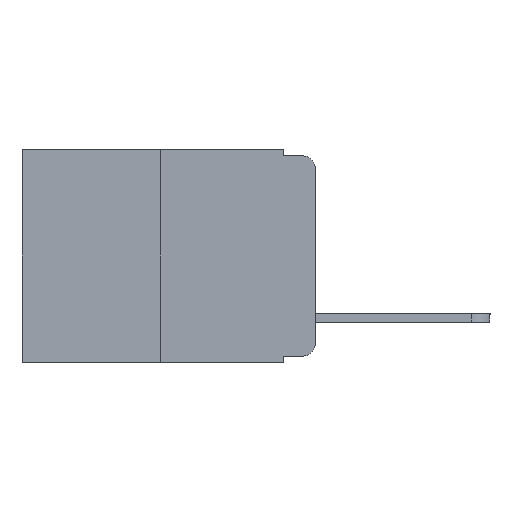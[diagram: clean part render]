
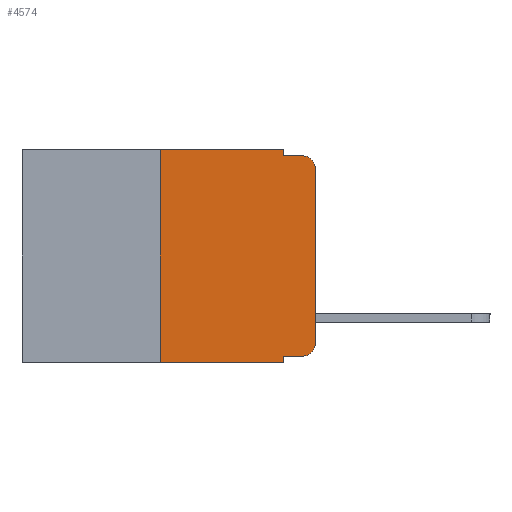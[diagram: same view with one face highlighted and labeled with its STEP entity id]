
A CAD part, left-side view. The second image highlights one B-rep face of the part: STEP entity #4574.
In plain terms, the highlighted planar face has unit normal (-1, 0, 0).
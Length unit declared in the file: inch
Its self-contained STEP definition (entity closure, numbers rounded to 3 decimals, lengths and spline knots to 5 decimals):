
#273 = VERTEX_POINT ( 'NONE', #12135 ) ;
#398 = VECTOR ( 'NONE', #12296, 39.37008 ) ;
#505 = CARTESIAN_POINT ( 'NONE',  ( 0., 0.051, 0. ) ) ;
#676 = EDGE_CURVE ( 'NONE', #2632, #12563, #696, .T. ) ;
#696 = LINE ( 'NONE', #2527, #10273 ) ;
#1191 = VERTEX_POINT ( 'NONE', #505 ) ;
#1200 = ORIENTED_EDGE ( 'NONE', *, *, #2599, .F. ) ;
#1659 = ORIENTED_EDGE ( 'NONE', *, *, #8141, .F. ) ;
#1666 = DIRECTION ( 'NONE',  ( 0., 0., -1. ) ) ;
#1713 = CARTESIAN_POINT ( 'NONE',  ( 0., 0.051, -0.333 ) ) ;
#2107 = VERTEX_POINT ( 'NONE', #7927 ) ;
#2180 = EDGE_CURVE ( 'NONE', #2632, #2240, #2536, .T. ) ;
#2240 = VERTEX_POINT ( 'NONE', #12593 ) ;
#2527 = CARTESIAN_POINT ( 'NONE',  ( 0., 0.051, -0.333 ) ) ;
#2536 = LINE ( 'NONE', #10856, #2968 ) ;
#2552 = EDGE_CURVE ( 'NONE', #2107, #11549, #4369, .T. ) ;
#2570 = DIRECTION ( 'NONE',  ( 0., -1., 0. ) ) ;
#2599 = EDGE_CURVE ( 'NONE', #1191, #11304, #6460, .T. ) ;
#2632 = VERTEX_POINT ( 'NONE', #1713 ) ;
#2968 = VECTOR ( 'NONE', #6342, 39.37008 ) ;
#3112 = LINE ( 'NONE', #13962, #9014 ) ;
#3216 = CARTESIAN_POINT ( 'NONE',  ( 0., 0.051, -0.01 ) ) ;
#3455 = EDGE_CURVE ( 'NONE', #273, #10642, #11468, .T. ) ;
#3740 = ORIENTED_EDGE ( 'NONE', *, *, #3455, .T. ) ;
#4049 = VERTEX_POINT ( 'NONE', #11626 ) ;
#4116 = CARTESIAN_POINT ( 'NONE',  ( 0., 0.02, -0.333 ) ) ;
#4196 = AXIS2_PLACEMENT_3D ( 'NONE', #6365, #13320, #7505 ) ;
#4369 = LINE ( 'NONE', #11781, #7522 ) ;
#4565 = EDGE_CURVE ( 'NONE', #10642, #4049, #13072, .T. ) ;
#4574 = ADVANCED_FACE ( 'NONE', ( #7935 ), #10622, .F. ) ;
#5543 = LINE ( 'NONE', #11296, #11242 ) ;
#5748 = EDGE_CURVE ( 'NONE', #11304, #4049, #3112, .T. ) ;
#5750 = DIRECTION ( 'NONE',  ( 0., -1., 0. ) ) ;
#6342 = DIRECTION ( 'NONE',  ( 0., 0., -1. ) ) ;
#6365 = CARTESIAN_POINT ( 'NONE',  ( 0., 0.02, -0.313 ) ) ;
#6460 = LINE ( 'NONE', #7733, #13944 ) ;
#6818 = ORIENTED_EDGE ( 'NONE', *, *, #5748, .F. ) ;
#7011 = ORIENTED_EDGE ( 'NONE', *, *, #676, .T. ) ;
#7505 = DIRECTION ( 'NONE',  ( 0., 0., -1. ) ) ;
#7522 = VECTOR ( 'NONE', #11786, 39.37008 ) ;
#7733 = CARTESIAN_POINT ( 'NONE',  ( 0., 0.051, 0. ) ) ;
#7927 = CARTESIAN_POINT ( 'NONE',  ( 0., 0.25, -0.343 ) ) ;
#7935 = FACE_OUTER_BOUND ( 'NONE', #11192, .T. ) ;
#8062 = ORIENTED_EDGE ( 'NONE', *, *, #10525, .T. ) ;
#8141 = EDGE_CURVE ( 'NONE', #11549, #1191, #5543, .T. ) ;
#8207 = EDGE_CURVE ( 'NONE', #2107, #2240, #12493, .T. ) ;
#8480 = AXIS2_PLACEMENT_3D ( 'NONE', #12536, #10586, #10603 ) ;
#8907 = ORIENTED_EDGE ( 'NONE', *, *, #8207, .T. ) ;
#9014 = VECTOR ( 'NONE', #10432, 39.37008 ) ;
#9222 = ORIENTED_EDGE ( 'NONE', *, *, #2180, .F. ) ;
#10180 = ORIENTED_EDGE ( 'NONE', *, *, #4565, .T. ) ;
#10273 = VECTOR ( 'NONE', #2570, 39.37008 ) ;
#10432 = DIRECTION ( 'NONE',  ( 0., -1., 0. ) ) ;
#10525 = EDGE_CURVE ( 'NONE', #12563, #273, #13809, .T. ) ;
#10586 = DIRECTION ( 'NONE',  ( -1., 0., 0. ) ) ;
#10603 = DIRECTION ( 'NONE',  ( 0., 0., -1. ) ) ;
#10622 = PLANE ( 'NONE',  #12953 ) ;
#10642 = VERTEX_POINT ( 'NONE', #12489 ) ;
#10856 = CARTESIAN_POINT ( 'NONE',  ( 0., 0.051, 0. ) ) ;
#11123 = DIRECTION ( 'NONE',  ( 1., 0., 0. ) ) ;
#11192 = EDGE_LOOP ( 'NONE', ( #3740, #10180, #6818, #1200, #1659, #11225, #8907, #9222, #7011, #8062 ) ) ;
#11225 = ORIENTED_EDGE ( 'NONE', *, *, #2552, .F. ) ;
#11242 = VECTOR ( 'NONE', #5750, 39.37008 ) ;
#11296 = CARTESIAN_POINT ( 'NONE',  ( 0., 0.473, 0. ) ) ;
#11304 = VERTEX_POINT ( 'NONE', #3216 ) ;
#11356 = CARTESIAN_POINT ( 'NONE',  ( 0., 0., 0. ) ) ;
#11386 = CARTESIAN_POINT ( 'NONE',  ( 0., 0.473, -0.343 ) ) ;
#11468 = LINE ( 'NONE', #11356, #13516 ) ;
#11549 = VERTEX_POINT ( 'NONE', #12157 ) ;
#11626 = CARTESIAN_POINT ( 'NONE',  ( 0., 0.02, -0.01 ) ) ;
#11781 = CARTESIAN_POINT ( 'NONE',  ( 0., 0.25, 0. ) ) ;
#11786 = DIRECTION ( 'NONE',  ( 0., 0., 1. ) ) ;
#12002 = DIRECTION ( 'NONE',  ( 0., 0., 1. ) ) ;
#12135 = CARTESIAN_POINT ( 'NONE',  ( 0., 0., -0.313 ) ) ;
#12157 = CARTESIAN_POINT ( 'NONE',  ( 0., 0.25, 0. ) ) ;
#12296 = DIRECTION ( 'NONE',  ( 0., -1., 0. ) ) ;
#12489 = CARTESIAN_POINT ( 'NONE',  ( 0., 0., -0.03 ) ) ;
#12493 = LINE ( 'NONE', #11386, #398 ) ;
#12495 = CARTESIAN_POINT ( 'NONE',  ( 0., 0.473, 0. ) ) ;
#12536 = CARTESIAN_POINT ( 'NONE',  ( 0., 0.02, -0.03 ) ) ;
#12563 = VERTEX_POINT ( 'NONE', #4116 ) ;
#12593 = CARTESIAN_POINT ( 'NONE',  ( 0., 0.051, -0.343 ) ) ;
#12953 = AXIS2_PLACEMENT_3D ( 'NONE', #12495, #11123, #1666 ) ;
#13071 = DIRECTION ( 'NONE',  ( 0., 0., -1. ) ) ;
#13072 = CIRCLE ( 'NONE', #8480, 0.02 ) ;
#13320 = DIRECTION ( 'NONE',  ( -1., 0., 0. ) ) ;
#13516 = VECTOR ( 'NONE', #12002, 39.37008 ) ;
#13809 = CIRCLE ( 'NONE', #4196, 0.02 ) ;
#13944 = VECTOR ( 'NONE', #13071, 39.37008 ) ;
#13962 = CARTESIAN_POINT ( 'NONE',  ( 0., 0.051, -0.01 ) ) ;
